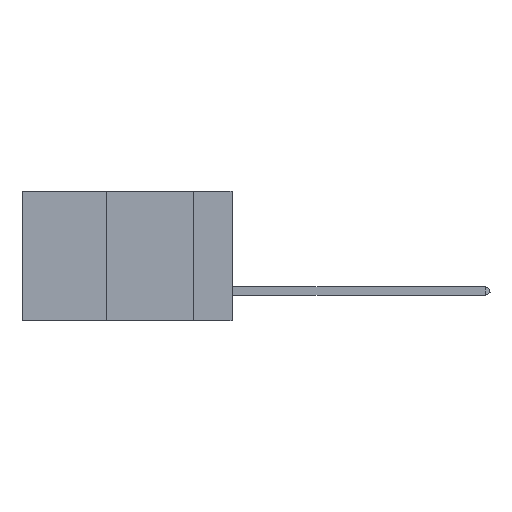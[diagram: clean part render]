
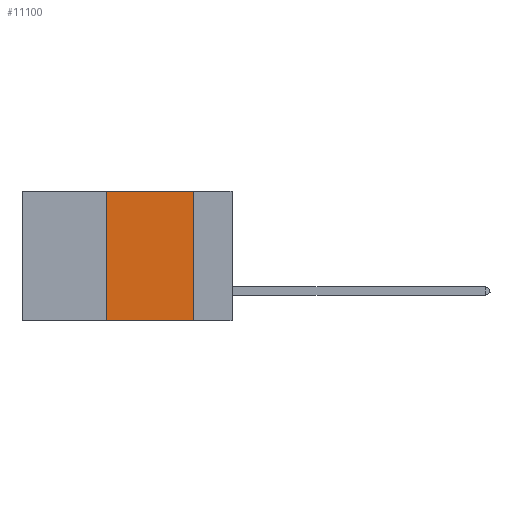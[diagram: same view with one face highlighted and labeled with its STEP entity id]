
A CAD part, left-side view. The second image highlights one B-rep face of the part: STEP entity #11100.
In plain terms, the highlighted planar face has unit normal (-1, 0, 0).
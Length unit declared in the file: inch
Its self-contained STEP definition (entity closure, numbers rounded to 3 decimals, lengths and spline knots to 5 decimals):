
#213 = CARTESIAN_POINT ( 'NONE',  ( 0., 0.36, -0.37 ) ) ;
#519 = DIRECTION ( 'NONE',  ( 1., 0., 0. ) ) ;
#1264 = VERTEX_POINT ( 'NONE', #213 ) ;
#1520 = ORIENTED_EDGE ( 'NONE', *, *, #17526, .F. ) ;
#2388 = EDGE_CURVE ( 'NONE', #7294, #13030, #8581, .T. ) ;
#2786 = VERTEX_POINT ( 'NONE', #16394 ) ;
#3614 = LINE ( 'NONE', #12600, #8369 ) ;
#4436 = LINE ( 'NONE', #6432, #15264 ) ;
#4913 = DIRECTION ( 'NONE',  ( 0., -1., 0. ) ) ;
#5846 = EDGE_CURVE ( 'NONE', #1264, #7294, #17159, .T. ) ;
#6432 = CARTESIAN_POINT ( 'NONE',  ( 0., 0.11, 0. ) ) ;
#6529 = ORIENTED_EDGE ( 'NONE', *, *, #2388, .F. ) ;
#7294 = VERTEX_POINT ( 'NONE', #16150 ) ;
#7751 = DIRECTION ( 'NONE',  ( 0., 0., -1. ) ) ;
#8261 = EDGE_CURVE ( 'NONE', #1264, #2786, #3614, .T. ) ;
#8369 = VECTOR ( 'NONE', #4913, 39.37008 ) ;
#8404 = FACE_OUTER_BOUND ( 'NONE', #9389, .T. ) ;
#8581 = LINE ( 'NONE', #17554, #14410 ) ;
#9389 = EDGE_LOOP ( 'NONE', ( #1520, #6529, #17417, #16693 ) ) ;
#9887 = AXIS2_PLACEMENT_3D ( 'NONE', #10379, #519, #10528 ) ;
#10379 = CARTESIAN_POINT ( 'NONE',  ( 0., 0.6, 0. ) ) ;
#10528 = DIRECTION ( 'NONE',  ( 0., 0., -1. ) ) ;
#11004 = DIRECTION ( 'NONE',  ( 0., -1., 0. ) ) ;
#11100 = ADVANCED_FACE ( 'NONE', ( #8404 ), #13729, .F. ) ;
#11917 = DIRECTION ( 'NONE',  ( 0., 0., 1. ) ) ;
#12600 = CARTESIAN_POINT ( 'NONE',  ( 0., 0.6, -0.37 ) ) ;
#12954 = VECTOR ( 'NONE', #11917, 39.37008 ) ;
#13030 = VERTEX_POINT ( 'NONE', #13521 ) ;
#13521 = CARTESIAN_POINT ( 'NONE',  ( 0., 0.11, 0. ) ) ;
#13729 = PLANE ( 'NONE',  #9887 ) ;
#14410 = VECTOR ( 'NONE', #11004, 39.37008 ) ;
#15264 = VECTOR ( 'NONE', #7751, 39.37008 ) ;
#16150 = CARTESIAN_POINT ( 'NONE',  ( 0., 0.36, 0. ) ) ;
#16394 = CARTESIAN_POINT ( 'NONE',  ( 0., 0.11, -0.37 ) ) ;
#16693 = ORIENTED_EDGE ( 'NONE', *, *, #8261, .T. ) ;
#16792 = CARTESIAN_POINT ( 'NONE',  ( 0., 0.36, 0. ) ) ;
#17159 = LINE ( 'NONE', #16792, #12954 ) ;
#17417 = ORIENTED_EDGE ( 'NONE', *, *, #5846, .F. ) ;
#17526 = EDGE_CURVE ( 'NONE', #13030, #2786, #4436, .T. ) ;
#17554 = CARTESIAN_POINT ( 'NONE',  ( 0., 0.6, 0. ) ) ;
